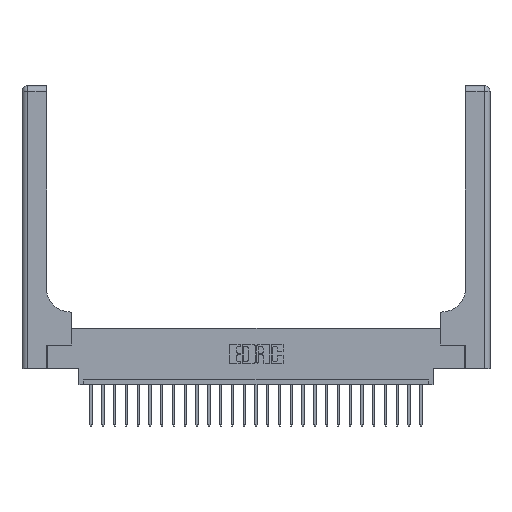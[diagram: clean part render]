
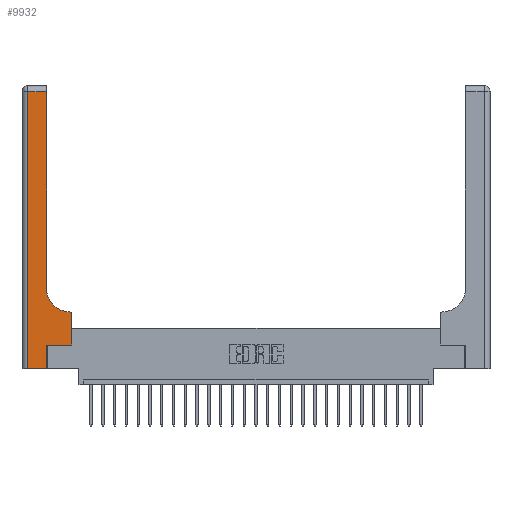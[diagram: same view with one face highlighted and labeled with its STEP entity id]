
A CAD part, top view. The second image highlights one B-rep face of the part: STEP entity #9932.
In plain terms, the highlighted planar face has unit normal (0, 0, 1).
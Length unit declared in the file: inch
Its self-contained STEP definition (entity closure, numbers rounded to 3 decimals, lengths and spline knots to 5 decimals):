
#108 = LINE ( 'NONE', #20553, #11689 ) ;
#315 = ORIENTED_EDGE ( 'NONE', *, *, #5434, .T. ) ;
#611 = CARTESIAN_POINT ( 'NONE',  ( 0.26, 2.94, 0.37 ) ) ;
#621 = CARTESIAN_POINT ( 'NONE',  ( 0.528, 0.25, 0.37 ) ) ;
#842 = VECTOR ( 'NONE', #15873, 39.37008 ) ;
#911 = EDGE_CURVE ( 'NONE', #16524, #5227, #21873, .T. ) ;
#1385 = FACE_OUTER_BOUND ( 'NONE', #24462, .T. ) ;
#1713 = CARTESIAN_POINT ( 'NONE',  ( 0.26, 0.6, 0.37 ) ) ;
#1971 = ORIENTED_EDGE ( 'NONE', *, *, #8981, .T. ) ;
#2065 = CARTESIAN_POINT ( 'NONE',  ( 0.265, 0., 0.37 ) ) ;
#2096 = CARTESIAN_POINT ( 'NONE',  ( 0.06, 3., 0.37 ) ) ;
#3279 = LINE ( 'NONE', #4571, #12114 ) ;
#3339 = VECTOR ( 'NONE', #16623, 39.37008 ) ;
#3666 = LINE ( 'NONE', #18564, #3339 ) ;
#4365 = LINE ( 'NONE', #24852, #6210 ) ;
#4534 = VERTEX_POINT ( 'NONE', #2065 ) ;
#4571 = CARTESIAN_POINT ( 'NONE',  ( 0., 0., 0.37 ) ) ;
#5227 = VERTEX_POINT ( 'NONE', #17917 ) ;
#5434 = EDGE_CURVE ( 'NONE', #18164, #16524, #4365, .T. ) ;
#5705 = DIRECTION ( 'NONE',  ( 0., 1., 0. ) ) ;
#6113 = ORIENTED_EDGE ( 'NONE', *, *, #11399, .T. ) ;
#6210 = VECTOR ( 'NONE', #5705, 39.37008 ) ;
#6925 = LINE ( 'NONE', #14275, #23855 ) ;
#7427 = EDGE_CURVE ( 'NONE', #8908, #17716, #3666, .T. ) ;
#7610 = DIRECTION ( 'NONE',  ( 1., 0., 0. ) ) ;
#8591 = CARTESIAN_POINT ( 'NONE',  ( 0., 3., 0.37 ) ) ;
#8674 = EDGE_CURVE ( 'NONE', #4534, #20590, #6925, .T. ) ;
#8908 = VERTEX_POINT ( 'NONE', #611 ) ;
#8981 = EDGE_CURVE ( 'NONE', #5227, #9635, #11706, .T. ) ;
#9082 = CARTESIAN_POINT ( 'NONE',  ( 0.51, 0.85, 0.37 ) ) ;
#9635 = VERTEX_POINT ( 'NONE', #24069 ) ;
#9932 = ADVANCED_FACE ( 'NONE', ( #1385 ), #16108, .F. ) ;
#10829 = ORIENTED_EDGE ( 'NONE', *, *, #23569, .T. ) ;
#11129 = ORIENTED_EDGE ( 'NONE', *, *, #23769, .T. ) ;
#11399 = EDGE_CURVE ( 'NONE', #20590, #18164, #19839, .T. ) ;
#11689 = VECTOR ( 'NONE', #22508, 39.37008 ) ;
#11706 = CIRCLE ( 'NONE', #20408, 0.25 ) ;
#12114 = VECTOR ( 'NONE', #12386, 39.37008 ) ;
#12141 = EDGE_CURVE ( 'NONE', #9635, #8908, #108, .T. ) ;
#12291 = VECTOR ( 'NONE', #21861, 39.37008 ) ;
#12344 = CARTESIAN_POINT ( 'NONE',  ( 0.265, 0.25, 0.37 ) ) ;
#12386 = DIRECTION ( 'NONE',  ( 1., 0., 0. ) ) ;
#13054 = ORIENTED_EDGE ( 'NONE', *, *, #8674, .T. ) ;
#14275 = CARTESIAN_POINT ( 'NONE',  ( 0.265, 0., 0.37 ) ) ;
#14423 = ORIENTED_EDGE ( 'NONE', *, *, #911, .T. ) ;
#15212 = DIRECTION ( 'NONE',  ( 0., 0., -1. ) ) ;
#15410 = CARTESIAN_POINT ( 'NONE',  ( 0.06, 0., 0.37 ) ) ;
#15873 = DIRECTION ( 'NONE',  ( 0., -1., 0. ) ) ;
#16108 = PLANE ( 'NONE',  #19272 ) ;
#16243 = DIRECTION ( 'NONE',  ( 0., 1., 0. ) ) ;
#16352 = CARTESIAN_POINT ( 'NONE',  ( 0.265, 0.25, 0.37 ) ) ;
#16355 = LINE ( 'NONE', #2096, #842 ) ;
#16451 = CARTESIAN_POINT ( 'NONE',  ( 0.06, 2.94, 0.37 ) ) ;
#16524 = VERTEX_POINT ( 'NONE', #17285 ) ;
#16623 = DIRECTION ( 'NONE',  ( -1., 0., 0. ) ) ;
#16832 = ORIENTED_EDGE ( 'NONE', *, *, #12141, .T. ) ;
#17285 = CARTESIAN_POINT ( 'NONE',  ( 0.528, 0.6, 0.37 ) ) ;
#17716 = VERTEX_POINT ( 'NONE', #16451 ) ;
#17917 = CARTESIAN_POINT ( 'NONE',  ( 0.51, 0.6, 0.37 ) ) ;
#18164 = VERTEX_POINT ( 'NONE', #621 ) ;
#18564 = CARTESIAN_POINT ( 'NONE',  ( 0., 2.94, 0.37 ) ) ;
#19126 = VERTEX_POINT ( 'NONE', #15410 ) ;
#19272 = AXIS2_PLACEMENT_3D ( 'NONE', #8591, #24086, #24178 ) ;
#19358 = ORIENTED_EDGE ( 'NONE', *, *, #7427, .T. ) ;
#19839 = LINE ( 'NONE', #12344, #12291 ) ;
#20408 = AXIS2_PLACEMENT_3D ( 'NONE', #9082, #15212, #7610 ) ;
#20553 = CARTESIAN_POINT ( 'NONE',  ( 0.26, 3., 0.37 ) ) ;
#20590 = VERTEX_POINT ( 'NONE', #16352 ) ;
#21861 = DIRECTION ( 'NONE',  ( 1., 0., 0. ) ) ;
#21873 = LINE ( 'NONE', #1713, #23404 ) ;
#22508 = DIRECTION ( 'NONE',  ( 0., 1., 0. ) ) ;
#22906 = DIRECTION ( 'NONE',  ( -1., 0., 0. ) ) ;
#23404 = VECTOR ( 'NONE', #22906, 39.37008 ) ;
#23569 = EDGE_CURVE ( 'NONE', #17716, #19126, #16355, .T. ) ;
#23769 = EDGE_CURVE ( 'NONE', #19126, #4534, #3279, .T. ) ;
#23855 = VECTOR ( 'NONE', #16243, 39.37008 ) ;
#24069 = CARTESIAN_POINT ( 'NONE',  ( 0.26, 0.85, 0.37 ) ) ;
#24086 = DIRECTION ( 'NONE',  ( 0., 0., -1. ) ) ;
#24178 = DIRECTION ( 'NONE',  ( -1., 0., 0. ) ) ;
#24462 = EDGE_LOOP ( 'NONE', ( #16832, #19358, #10829, #11129, #13054, #6113, #315, #14423, #1971 ) ) ;
#24852 = CARTESIAN_POINT ( 'NONE',  ( 0.528, 0.25, 0.37 ) ) ;
